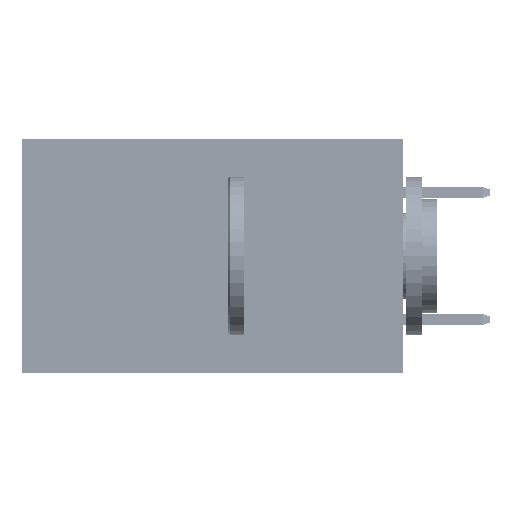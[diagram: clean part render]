
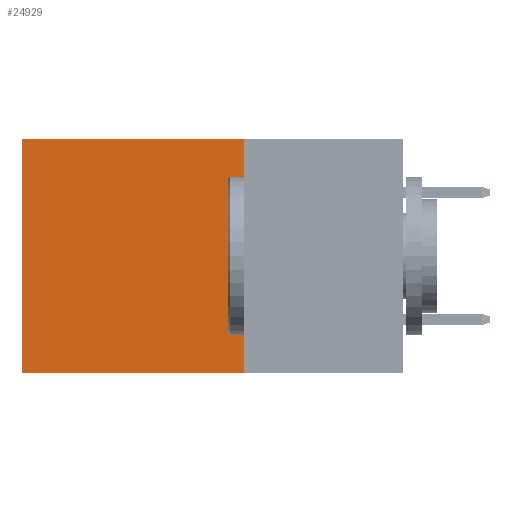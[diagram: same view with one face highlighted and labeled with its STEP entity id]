
A CAD part, left-side view. The second image highlights one B-rep face of the part: STEP entity #24929.
In plain terms, the highlighted planar face has unit normal (-1, 0, 0).
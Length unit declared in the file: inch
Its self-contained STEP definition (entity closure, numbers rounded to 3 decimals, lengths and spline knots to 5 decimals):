
#704 = EDGE_CURVE ( 'NONE', #36715, #40920, #43795, .T. ) ;
#2365 = LINE ( 'NONE', #33639, #42954 ) ;
#2652 = CARTESIAN_POINT ( 'NONE',  ( 0.2875, 0.6, 0. ) ) ;
#9910 = ORIENTED_EDGE ( 'NONE', *, *, #28810, .F. ) ;
#10335 = DIRECTION ( 'NONE',  ( 0., 1., 0. ) ) ;
#10425 = CARTESIAN_POINT ( 'NONE',  ( 0.2875, 0.6, -0.37 ) ) ;
#12890 = DIRECTION ( 'NONE',  ( 0., 0., -1. ) ) ;
#12933 = EDGE_CURVE ( 'NONE', #36715, #19747, #17244, .T. ) ;
#13224 = AXIS2_PLACEMENT_3D ( 'NONE', #48170, #21040, #37168 ) ;
#13294 = CARTESIAN_POINT ( 'NONE',  ( 0.2875, 0.25, 0. ) ) ;
#17244 = LINE ( 'NONE', #36222, #24895 ) ;
#17435 = PLANE ( 'NONE',  #13224 ) ;
#19747 = VERTEX_POINT ( 'NONE', #35016 ) ;
#21040 = DIRECTION ( 'NONE',  ( 1., 0., 0. ) ) ;
#24563 = CARTESIAN_POINT ( 'NONE',  ( 0.2875, 0.25, 0. ) ) ;
#24895 = VECTOR ( 'NONE', #12890, 39.37008 ) ;
#24929 = ADVANCED_FACE ( 'NONE', ( #32566 ), #17435, .F. ) ;
#28686 = DIRECTION ( 'NONE',  ( 0., 1., 0. ) ) ;
#28810 = EDGE_CURVE ( 'NONE', #19747, #31454, #2365, .T. ) ;
#29603 = LINE ( 'NONE', #33456, #36035 ) ;
#30877 = ORIENTED_EDGE ( 'NONE', *, *, #12933, .F. ) ;
#31276 = EDGE_LOOP ( 'NONE', ( #35213, #9910, #30877, #41282 ) ) ;
#31454 = VERTEX_POINT ( 'NONE', #10425 ) ;
#32566 = FACE_OUTER_BOUND ( 'NONE', #31276, .T. ) ;
#33456 = CARTESIAN_POINT ( 'NONE',  ( 0.2875, 0.6, 0. ) ) ;
#33639 = CARTESIAN_POINT ( 'NONE',  ( 0.2875, 0.25, -0.37 ) ) ;
#35016 = CARTESIAN_POINT ( 'NONE',  ( 0.2875, 0.25, -0.37 ) ) ;
#35213 = ORIENTED_EDGE ( 'NONE', *, *, #45159, .T. ) ;
#36035 = VECTOR ( 'NONE', #41655, 39.37008 ) ;
#36222 = CARTESIAN_POINT ( 'NONE',  ( 0.2875, 0.25, 0. ) ) ;
#36380 = VECTOR ( 'NONE', #28686, 39.37008 ) ;
#36715 = VERTEX_POINT ( 'NONE', #24563 ) ;
#37168 = DIRECTION ( 'NONE',  ( 0., 0., -1. ) ) ;
#40920 = VERTEX_POINT ( 'NONE', #2652 ) ;
#41282 = ORIENTED_EDGE ( 'NONE', *, *, #704, .T. ) ;
#41655 = DIRECTION ( 'NONE',  ( 0., 0., -1. ) ) ;
#42954 = VECTOR ( 'NONE', #10335, 39.37008 ) ;
#43795 = LINE ( 'NONE', #13294, #36380 ) ;
#45159 = EDGE_CURVE ( 'NONE', #40920, #31454, #29603, .T. ) ;
#48170 = CARTESIAN_POINT ( 'NONE',  ( 0.2875, 0.25, 0. ) ) ;
